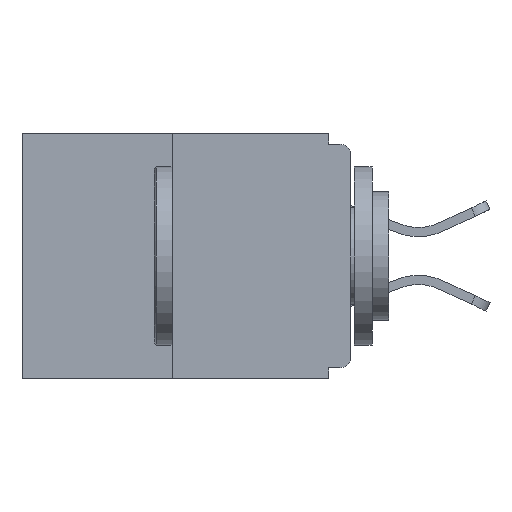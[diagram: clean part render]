
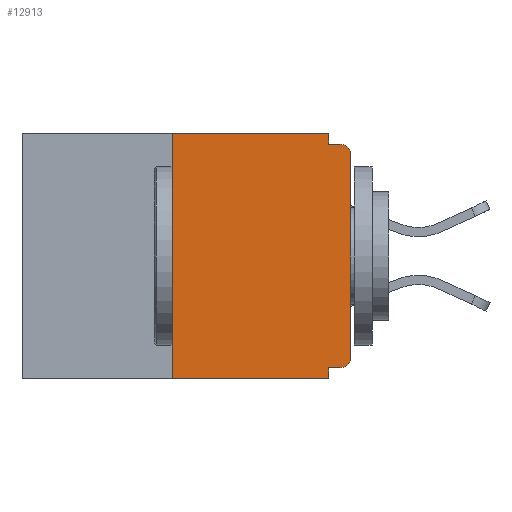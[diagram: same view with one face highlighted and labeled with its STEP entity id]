
A CAD part, left-side view. The second image highlights one B-rep face of the part: STEP entity #12913.
In plain terms, the highlighted planar face has unit normal (-1, 0, 0).
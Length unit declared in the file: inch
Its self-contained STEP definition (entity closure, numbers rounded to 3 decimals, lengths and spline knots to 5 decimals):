
#169 = VECTOR ( 'NONE', #1691, 39.37008 ) ;
#868 = EDGE_CURVE ( 'NONE', #6983, #5504, #8901, .T. ) ;
#916 = CARTESIAN_POINT ( 'NONE',  ( 0., 0.25, 0. ) ) ;
#1020 = CARTESIAN_POINT ( 'NONE',  ( 0., 0.031, -0.328 ) ) ;
#1691 = DIRECTION ( 'NONE',  ( 0., 1., 0. ) ) ;
#1721 = CARTESIAN_POINT ( 'NONE',  ( 0., 0.46, 0. ) ) ;
#1764 = EDGE_CURVE ( 'NONE', #14078, #13862, #9590, .T. ) ;
#1902 = VECTOR ( 'NONE', #9969, 39.37008 ) ;
#1979 = LINE ( 'NONE', #7573, #169 ) ;
#2069 = LINE ( 'NONE', #2151, #11496 ) ;
#2151 = CARTESIAN_POINT ( 'NONE',  ( 0., 0., -0.015 ) ) ;
#2227 = LINE ( 'NONE', #5450, #2396 ) ;
#2396 = VECTOR ( 'NONE', #10298, 39.37008 ) ;
#2617 = CARTESIAN_POINT ( 'NONE',  ( 0., 0.015, -0.015 ) ) ;
#2664 = ORIENTED_EDGE ( 'NONE', *, *, #9649, .F. ) ;
#2903 = CARTESIAN_POINT ( 'NONE',  ( 0., 0.031, -0.343 ) ) ;
#3645 = CARTESIAN_POINT ( 'NONE',  ( 0., 0.031, -0.343 ) ) ;
#3864 = ORIENTED_EDGE ( 'NONE', *, *, #5859, .T. ) ;
#4087 = EDGE_LOOP ( 'NONE', ( #12377, #14988, #10547, #12122, #4942, #13840, #3864, #5503, #2664, #10797 ) ) ;
#4575 = CIRCLE ( 'NONE', #8644, 0.015 ) ;
#4831 = AXIS2_PLACEMENT_3D ( 'NONE', #1721, #13498, #14727 ) ;
#4933 = CARTESIAN_POINT ( 'NONE',  ( 0., 0., 0. ) ) ;
#4942 = ORIENTED_EDGE ( 'NONE', *, *, #12641, .F. ) ;
#5353 = VERTEX_POINT ( 'NONE', #5984 ) ;
#5450 = CARTESIAN_POINT ( 'NONE',  ( 0., 0.25, 0. ) ) ;
#5503 = ORIENTED_EDGE ( 'NONE', *, *, #1764, .T. ) ;
#5504 = VERTEX_POINT ( 'NONE', #6292 ) ;
#5588 = EDGE_CURVE ( 'NONE', #5504, #5353, #14261, .T. ) ;
#5859 = EDGE_CURVE ( 'NONE', #10336, #14078, #12230, .T. ) ;
#5984 = CARTESIAN_POINT ( 'NONE',  ( 0., 0.031, -0.015 ) ) ;
#6292 = CARTESIAN_POINT ( 'NONE',  ( 0., 0.031, 0. ) ) ;
#6517 = DIRECTION ( 'NONE',  ( -1., 0., 0. ) ) ;
#6784 = LINE ( 'NONE', #8381, #14010 ) ;
#6974 = DIRECTION ( 'NONE',  ( 0., 0., -1. ) ) ;
#6983 = VERTEX_POINT ( 'NONE', #916 ) ;
#7451 = AXIS2_PLACEMENT_3D ( 'NONE', #12817, #12764, #6974 ) ;
#7573 = CARTESIAN_POINT ( 'NONE',  ( 0., 0., -0.328 ) ) ;
#7669 = DIRECTION ( 'NONE',  ( 0., 0., -1. ) ) ;
#8006 = DIRECTION ( 'NONE',  ( 0., -1., 0. ) ) ;
#8099 = VERTEX_POINT ( 'NONE', #9631 ) ;
#8344 = VERTEX_POINT ( 'NONE', #3645 ) ;
#8381 = CARTESIAN_POINT ( 'NONE',  ( 0., 0.46, -0.343 ) ) ;
#8644 = AXIS2_PLACEMENT_3D ( 'NONE', #13419, #6517, #7669 ) ;
#8700 = CARTESIAN_POINT ( 'NONE',  ( 0., 0.46, 0. ) ) ;
#8873 = PLANE ( 'NONE',  #4831 ) ;
#8901 = LINE ( 'NONE', #8700, #9978 ) ;
#9590 = CIRCLE ( 'NONE', #7451, 0.015 ) ;
#9599 = VERTEX_POINT ( 'NONE', #1020 ) ;
#9631 = CARTESIAN_POINT ( 'NONE',  ( 0., 0.015, -0.328 ) ) ;
#9649 = EDGE_CURVE ( 'NONE', #5353, #13862, #2069, .T. ) ;
#9969 = DIRECTION ( 'NONE',  ( 0., 0., -1. ) ) ;
#9978 = VECTOR ( 'NONE', #14493, 39.37008 ) ;
#10071 = VECTOR ( 'NONE', #13047, 39.37008 ) ;
#10160 = EDGE_CURVE ( 'NONE', #12001, #6983, #2227, .T. ) ;
#10298 = DIRECTION ( 'NONE',  ( 0., 0., 1. ) ) ;
#10329 = FACE_OUTER_BOUND ( 'NONE', #4087, .T. ) ;
#10336 = VERTEX_POINT ( 'NONE', #13175 ) ;
#10547 = ORIENTED_EDGE ( 'NONE', *, *, #11630, .T. ) ;
#10563 = EDGE_CURVE ( 'NONE', #8099, #10336, #4575, .T. ) ;
#10708 = VECTOR ( 'NONE', #12193, 39.37008 ) ;
#10797 = ORIENTED_EDGE ( 'NONE', *, *, #5588, .F. ) ;
#11496 = VECTOR ( 'NONE', #8006, 39.37008 ) ;
#11630 = EDGE_CURVE ( 'NONE', #12001, #8344, #6784, .T. ) ;
#12001 = VERTEX_POINT ( 'NONE', #13048 ) ;
#12122 = ORIENTED_EDGE ( 'NONE', *, *, #12674, .F. ) ;
#12193 = DIRECTION ( 'NONE',  ( 0., 0., -1. ) ) ;
#12230 = LINE ( 'NONE', #4933, #10071 ) ;
#12348 = CARTESIAN_POINT ( 'NONE',  ( 0., 0., -0.03 ) ) ;
#12377 = ORIENTED_EDGE ( 'NONE', *, *, #868, .F. ) ;
#12641 = EDGE_CURVE ( 'NONE', #8099, #9599, #1979, .T. ) ;
#12674 = EDGE_CURVE ( 'NONE', #9599, #8344, #13795, .T. ) ;
#12764 = DIRECTION ( 'NONE',  ( -1., 0., 0. ) ) ;
#12817 = CARTESIAN_POINT ( 'NONE',  ( 0., 0.015, -0.03 ) ) ;
#12913 = ADVANCED_FACE ( 'NONE', ( #10329 ), #8873, .F. ) ;
#12926 = DIRECTION ( 'NONE',  ( 0., -1., 0. ) ) ;
#13047 = DIRECTION ( 'NONE',  ( 0., 0., 1. ) ) ;
#13048 = CARTESIAN_POINT ( 'NONE',  ( 0., 0.25, -0.343 ) ) ;
#13175 = CARTESIAN_POINT ( 'NONE',  ( 0., 0., -0.313 ) ) ;
#13419 = CARTESIAN_POINT ( 'NONE',  ( 0., 0.015, -0.313 ) ) ;
#13452 = CARTESIAN_POINT ( 'NONE',  ( 0., 0.031, 0. ) ) ;
#13498 = DIRECTION ( 'NONE',  ( 1., 0., 0. ) ) ;
#13795 = LINE ( 'NONE', #2903, #10708 ) ;
#13840 = ORIENTED_EDGE ( 'NONE', *, *, #10563, .T. ) ;
#13862 = VERTEX_POINT ( 'NONE', #2617 ) ;
#14010 = VECTOR ( 'NONE', #12926, 39.37008 ) ;
#14078 = VERTEX_POINT ( 'NONE', #12348 ) ;
#14261 = LINE ( 'NONE', #13452, #1902 ) ;
#14493 = DIRECTION ( 'NONE',  ( 0., -1., 0. ) ) ;
#14727 = DIRECTION ( 'NONE',  ( 0., 0., -1. ) ) ;
#14988 = ORIENTED_EDGE ( 'NONE', *, *, #10160, .F. ) ;
